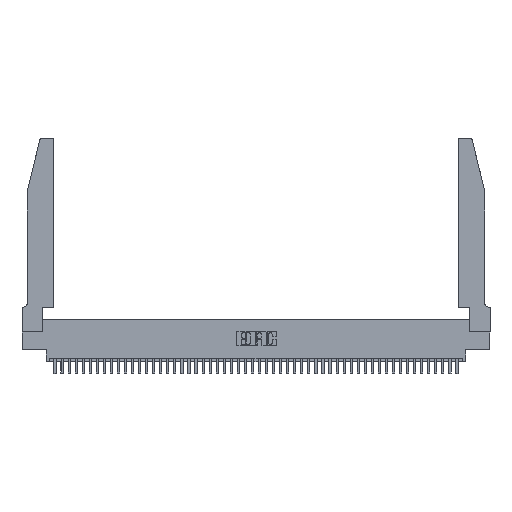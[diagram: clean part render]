
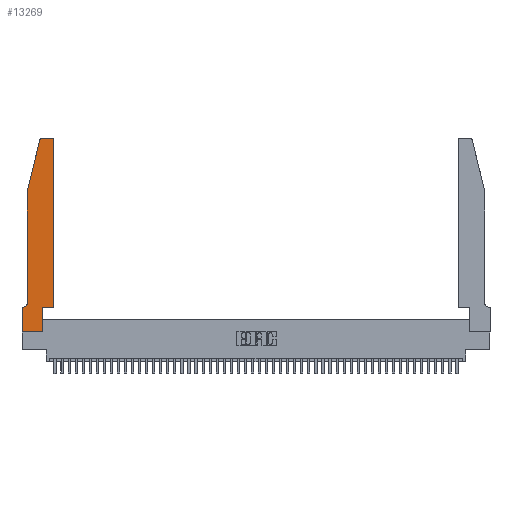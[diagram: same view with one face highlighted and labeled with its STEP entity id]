
A CAD part, top view. The second image highlights one B-rep face of the part: STEP entity #13269.
In plain terms, the highlighted planar face has unit normal (0, 0, 1).
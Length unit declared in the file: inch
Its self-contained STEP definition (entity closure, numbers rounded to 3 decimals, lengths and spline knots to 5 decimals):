
#51 = CARTESIAN_POINT ( 'NONE',  ( 0.284, 2.75, 0.37 ) ) ;
#213 = DIRECTION ( 'NONE',  ( 1., 0., 0. ) ) ;
#465 = ORIENTED_EDGE ( 'NONE', *, *, #7933, .T. ) ;
#496 = VERTEX_POINT ( 'NONE', #37918 ) ;
#626 = LINE ( 'NONE', #8755, #9360 ) ;
#1368 = EDGE_CURVE ( 'NONE', #45397, #29795, #26841, .T. ) ;
#1598 = CARTESIAN_POINT ( 'NONE',  ( 0.4505, 2.72, 0.37 ) ) ;
#1751 = EDGE_CURVE ( 'NONE', #37056, #27279, #39071, .T. ) ;
#2104 = CARTESIAN_POINT ( 'NONE',  ( 0., 0.35, 0.37 ) ) ;
#2188 = EDGE_CURVE ( 'NONE', #47098, #14544, #31472, .T. ) ;
#3144 = CARTESIAN_POINT ( 'NONE',  ( 0.2605, 2.75, 0.37 ) ) ;
#3844 = CARTESIAN_POINT ( 'NONE',  ( 0., 0., 0.37 ) ) ;
#3935 = CARTESIAN_POINT ( 'NONE',  ( 0.25487, 2.72718, 0.37 ) ) ;
#3972 = DIRECTION ( 'NONE',  ( 0., 0., 1. ) ) ;
#4270 = EDGE_CURVE ( 'NONE', #13334, #37056, #4478, .T. ) ;
#4478 = LINE ( 'NONE', #37490, #14324 ) ;
#4538 = AXIS2_PLACEMENT_3D ( 'NONE', #43521, #21078, #47326 ) ;
#4922 = CARTESIAN_POINT ( 'NONE',  ( 0., 0., 0.37 ) ) ;
#5059 = ORIENTED_EDGE ( 'NONE', *, *, #4270, .T. ) ;
#5359 = CARTESIAN_POINT ( 'NONE',  ( 0.2865, 0.35, 0.37 ) ) ;
#5443 = ORIENTED_EDGE ( 'NONE', *, *, #34745, .T. ) ;
#5601 = VECTOR ( 'NONE', #19920, 39.37008 ) ;
#6755 = LINE ( 'NONE', #38482, #5601 ) ;
#7754 = CARTESIAN_POINT ( 'NONE',  ( 0.4505, 0.35, 0.37 ) ) ;
#7933 = EDGE_CURVE ( 'NONE', #10999, #40910, #626, .T. ) ;
#8755 = CARTESIAN_POINT ( 'NONE',  ( 0.2865, 0.35, 0.37 ) ) ;
#9233 = ORIENTED_EDGE ( 'NONE', *, *, #31800, .T. ) ;
#9360 = VECTOR ( 'NONE', #42329, 39.37008 ) ;
#9408 = CARTESIAN_POINT ( 'NONE',  ( 0.4505, 0.35, 0.37 ) ) ;
#9426 = VECTOR ( 'NONE', #19110, 39.37008 ) ;
#10999 = VERTEX_POINT ( 'NONE', #30083 ) ;
#11885 = ORIENTED_EDGE ( 'NONE', *, *, #1751, .T. ) ;
#13269 = ADVANCED_FACE ( 'NONE', ( #36799 ), #48188, .T. ) ;
#13334 = VERTEX_POINT ( 'NONE', #3935 ) ;
#13488 = DIRECTION ( 'NONE',  ( -1., 0., 0. ) ) ;
#14324 = VECTOR ( 'NONE', #30014, 39.37008 ) ;
#14544 = VERTEX_POINT ( 'NONE', #28745 ) ;
#14585 = EDGE_CURVE ( 'NONE', #14544, #41349, #18028, .T. ) ;
#15717 = CARTESIAN_POINT ( 'NONE',  ( 0.0055, 0.42, 0.37 ) ) ;
#15752 = VECTOR ( 'NONE', #27078, 39.37008 ) ;
#16996 = VECTOR ( 'NONE', #13488, 39.37008 ) ;
#18028 = LINE ( 'NONE', #3144, #27887 ) ;
#18335 = DIRECTION ( 'NONE',  ( 1., 0., 0. ) ) ;
#19110 = DIRECTION ( 'NONE',  ( 0., -1., 0. ) ) ;
#19433 = DIRECTION ( 'NONE',  ( -1., 0., 0. ) ) ;
#19920 = DIRECTION ( 'NONE',  ( 1., 0., 0. ) ) ;
#21078 = DIRECTION ( 'NONE',  ( 0., 0., 1. ) ) ;
#21300 = ORIENTED_EDGE ( 'NONE', *, *, #27236, .T. ) ;
#22328 = ORIENTED_EDGE ( 'NONE', *, *, #29667, .T. ) ;
#22402 = AXIS2_PLACEMENT_3D ( 'NONE', #26146, #3972, #29901 ) ;
#22648 = ORIENTED_EDGE ( 'NONE', *, *, #36436, .T. ) ;
#26146 = CARTESIAN_POINT ( 'NONE',  ( 0.284, 2.72, 0.37 ) ) ;
#26841 = LINE ( 'NONE', #39511, #16996 ) ;
#27078 = DIRECTION ( 'NONE',  ( 0., -1., 0. ) ) ;
#27236 = EDGE_CURVE ( 'NONE', #27279, #45397, #37263, .T. ) ;
#27279 = VERTEX_POINT ( 'NONE', #30848 ) ;
#27401 = ORIENTED_EDGE ( 'NONE', *, *, #2188, .T. ) ;
#27887 = VECTOR ( 'NONE', #29075, 39.37008 ) ;
#28745 = CARTESIAN_POINT ( 'NONE',  ( 0.4205, 2.75, 0.37 ) ) ;
#29075 = DIRECTION ( 'NONE',  ( -1., 0., 0. ) ) ;
#29667 = EDGE_CURVE ( 'NONE', #40910, #35155, #6755, .T. ) ;
#29795 = VERTEX_POINT ( 'NONE', #2104 ) ;
#29901 = DIRECTION ( 'NONE',  ( 1., 0., 0. ) ) ;
#30014 = DIRECTION ( 'NONE',  ( -0.239, -0.971, 0. ) ) ;
#30045 = ORIENTED_EDGE ( 'NONE', *, *, #14585, .T. ) ;
#30083 = CARTESIAN_POINT ( 'NONE',  ( 0.2865, 0., 0.37 ) ) ;
#30345 = CARTESIAN_POINT ( 'NONE',  ( 0.0755, 2., 0.37 ) ) ;
#30848 = CARTESIAN_POINT ( 'NONE',  ( 0.0755, 0.42, 0.37 ) ) ;
#31072 = LINE ( 'NONE', #9408, #32244 ) ;
#31472 = CIRCLE ( 'NONE', #4538, 0.03 ) ;
#31800 = EDGE_CURVE ( 'NONE', #41349, #13334, #43274, .T. ) ;
#31968 = ORIENTED_EDGE ( 'NONE', *, *, #41377, .T. ) ;
#32244 = VECTOR ( 'NONE', #35386, 39.37008 ) ;
#34745 = EDGE_CURVE ( 'NONE', #35155, #47098, #31072, .T. ) ;
#35155 = VERTEX_POINT ( 'NONE', #7754 ) ;
#35386 = DIRECTION ( 'NONE',  ( 0., 1., 0. ) ) ;
#36436 = EDGE_CURVE ( 'NONE', #29795, #496, #44438, .T. ) ;
#36799 = FACE_OUTER_BOUND ( 'NONE', #44169, .T. ) ;
#36883 = CARTESIAN_POINT ( 'NONE',  ( 0., 0.35, 0.37 ) ) ;
#37056 = VERTEX_POINT ( 'NONE', #45788 ) ;
#37141 = AXIS2_PLACEMENT_3D ( 'NONE', #36883, #40689, #18335 ) ;
#37263 = CIRCLE ( 'NONE', #40443, 0.07 ) ;
#37490 = CARTESIAN_POINT ( 'NONE',  ( 0.0755, 2., 0.37 ) ) ;
#37506 = LINE ( 'NONE', #3844, #47646 ) ;
#37918 = CARTESIAN_POINT ( 'NONE',  ( 0., 0., 0.37 ) ) ;
#38300 = CARTESIAN_POINT ( 'NONE',  ( 0.0055, 0.35, 0.37 ) ) ;
#38482 = CARTESIAN_POINT ( 'NONE',  ( 0.4505, 0.35, 0.37 ) ) ;
#39071 = LINE ( 'NONE', #30345, #9426 ) ;
#39511 = CARTESIAN_POINT ( 'NONE',  ( 0.0755, 0.35, 0.37 ) ) ;
#40443 = AXIS2_PLACEMENT_3D ( 'NONE', #15717, #41834, #19433 ) ;
#40689 = DIRECTION ( 'NONE',  ( 0., 0., 1. ) ) ;
#40910 = VERTEX_POINT ( 'NONE', #5359 ) ;
#41349 = VERTEX_POINT ( 'NONE', #51 ) ;
#41377 = EDGE_CURVE ( 'NONE', #496, #10999, #37506, .T. ) ;
#41834 = DIRECTION ( 'NONE',  ( 0., 0., -1. ) ) ;
#42329 = DIRECTION ( 'NONE',  ( 0., 1., 0. ) ) ;
#43274 = CIRCLE ( 'NONE', #22402, 0.03 ) ;
#43521 = CARTESIAN_POINT ( 'NONE',  ( 0.4205, 2.72, 0.37 ) ) ;
#44169 = EDGE_LOOP ( 'NONE', ( #30045, #9233, #5059, #11885, #21300, #46829, #22648, #31968, #465, #22328, #5443, #27401 ) ) ;
#44438 = LINE ( 'NONE', #4922, #15752 ) ;
#45397 = VERTEX_POINT ( 'NONE', #38300 ) ;
#45788 = CARTESIAN_POINT ( 'NONE',  ( 0.0755, 2., 0.37 ) ) ;
#46829 = ORIENTED_EDGE ( 'NONE', *, *, #1368, .T. ) ;
#47098 = VERTEX_POINT ( 'NONE', #1598 ) ;
#47326 = DIRECTION ( 'NONE',  ( 1., 0., 0. ) ) ;
#47646 = VECTOR ( 'NONE', #213, 39.37008 ) ;
#48188 = PLANE ( 'NONE',  #37141 ) ;
